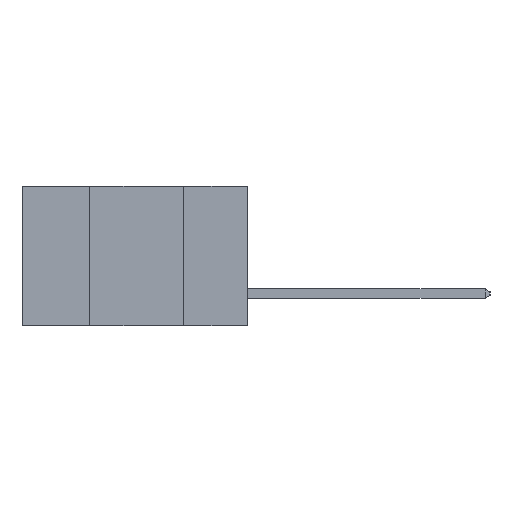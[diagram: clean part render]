
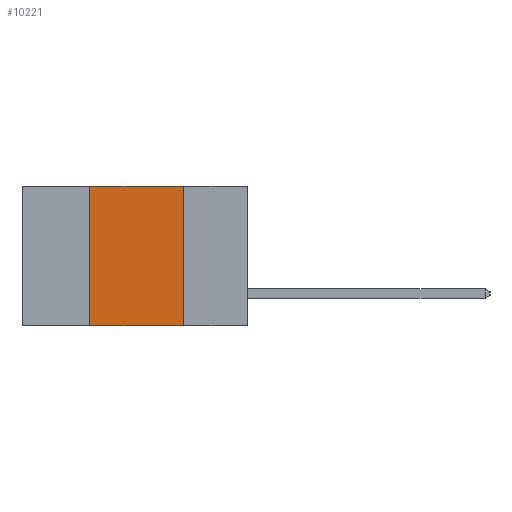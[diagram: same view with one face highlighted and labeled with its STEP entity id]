
A CAD part, left-side view. The second image highlights one B-rep face of the part: STEP entity #10221.
In plain terms, the highlighted planar face has unit normal (-1, 0, 0).
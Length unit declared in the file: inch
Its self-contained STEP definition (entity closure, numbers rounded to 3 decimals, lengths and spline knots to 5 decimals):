
#333 = VERTEX_POINT ( 'NONE', #3176 ) ;
#1209 = CARTESIAN_POINT ( 'NONE',  ( 0., 0.6, -0.37 ) ) ;
#2687 = ORIENTED_EDGE ( 'NONE', *, *, #15561, .F. ) ;
#2758 = EDGE_LOOP ( 'NONE', ( #16803, #2687, #6965, #14897 ) ) ;
#3176 = CARTESIAN_POINT ( 'NONE',  ( 0., 0.42, -0.37 ) ) ;
#3286 = LINE ( 'NONE', #13703, #10374 ) ;
#3745 = LINE ( 'NONE', #16629, #7053 ) ;
#3758 = DIRECTION ( 'NONE',  ( 1., 0., 0. ) ) ;
#3834 = VECTOR ( 'NONE', #12742, 39.37008 ) ;
#4137 = VECTOR ( 'NONE', #8849, 39.37008 ) ;
#4267 = LINE ( 'NONE', #1209, #3834 ) ;
#4348 = EDGE_CURVE ( 'NONE', #5151, #15491, #3286, .T. ) ;
#5151 = VERTEX_POINT ( 'NONE', #5774 ) ;
#5774 = CARTESIAN_POINT ( 'NONE',  ( 0., 0.17, 0. ) ) ;
#6965 = ORIENTED_EDGE ( 'NONE', *, *, #14743, .F. ) ;
#7053 = VECTOR ( 'NONE', #9667, 39.37008 ) ;
#7775 = EDGE_CURVE ( 'NONE', #333, #15491, #4267, .T. ) ;
#8849 = DIRECTION ( 'NONE',  ( 0., -1., 0. ) ) ;
#9667 = DIRECTION ( 'NONE',  ( 0., 0., 1. ) ) ;
#10221 = ADVANCED_FACE ( 'NONE', ( #14494 ), #17696, .F. ) ;
#10374 = VECTOR ( 'NONE', #13554, 39.37008 ) ;
#12224 = CARTESIAN_POINT ( 'NONE',  ( 0., 0.6, 0. ) ) ;
#12503 = AXIS2_PLACEMENT_3D ( 'NONE', #12224, #3758, #13650 ) ;
#12742 = DIRECTION ( 'NONE',  ( 0., -1., 0. ) ) ;
#12942 = CARTESIAN_POINT ( 'NONE',  ( 0., 0.17, -0.37 ) ) ;
#13554 = DIRECTION ( 'NONE',  ( 0., 0., -1. ) ) ;
#13650 = DIRECTION ( 'NONE',  ( 0., 0., -1. ) ) ;
#13703 = CARTESIAN_POINT ( 'NONE',  ( 0., 0.17, 0. ) ) ;
#14141 = VERTEX_POINT ( 'NONE', #15707 ) ;
#14494 = FACE_OUTER_BOUND ( 'NONE', #2758, .T. ) ;
#14743 = EDGE_CURVE ( 'NONE', #333, #14141, #3745, .T. ) ;
#14897 = ORIENTED_EDGE ( 'NONE', *, *, #7775, .T. ) ;
#15349 = LINE ( 'NONE', #17202, #4137 ) ;
#15491 = VERTEX_POINT ( 'NONE', #12942 ) ;
#15561 = EDGE_CURVE ( 'NONE', #14141, #5151, #15349, .T. ) ;
#15707 = CARTESIAN_POINT ( 'NONE',  ( 0., 0.42, 0. ) ) ;
#16629 = CARTESIAN_POINT ( 'NONE',  ( 0., 0.42, 0. ) ) ;
#16803 = ORIENTED_EDGE ( 'NONE', *, *, #4348, .F. ) ;
#17202 = CARTESIAN_POINT ( 'NONE',  ( 0., 0.6, 0. ) ) ;
#17696 = PLANE ( 'NONE',  #12503 ) ;
